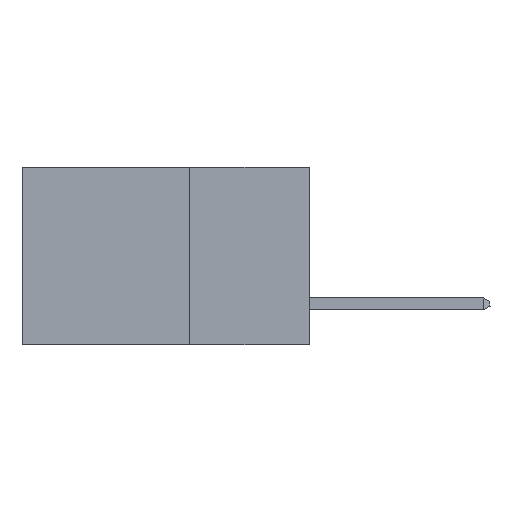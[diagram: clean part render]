
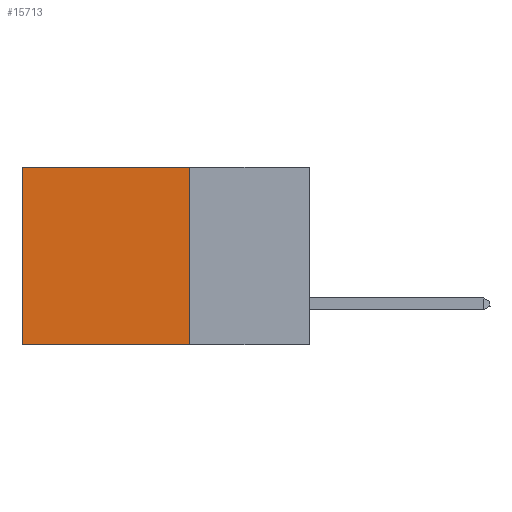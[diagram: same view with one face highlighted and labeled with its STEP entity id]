
A CAD part, left-side view. The second image highlights one B-rep face of the part: STEP entity #15713.
In plain terms, the highlighted planar face has unit normal (-1, 0, 0).
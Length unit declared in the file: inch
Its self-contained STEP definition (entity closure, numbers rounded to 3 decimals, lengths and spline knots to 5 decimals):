
#257 = VERTEX_POINT ( 'NONE', #1557 ) ;
#880 = LINE ( 'NONE', #9401, #15847 ) ;
#1231 = VERTEX_POINT ( 'NONE', #15142 ) ;
#1557 = CARTESIAN_POINT ( 'NONE',  ( 0.2875, 0.6, -0.37 ) ) ;
#1812 = CARTESIAN_POINT ( 'NONE',  ( 0.2875, 0.25, 0. ) ) ;
#1836 = CARTESIAN_POINT ( 'NONE',  ( 0.2875, 0.25, 0. ) ) ;
#1911 = VECTOR ( 'NONE', #5494, 39.37008 ) ;
#2403 = DIRECTION ( 'NONE',  ( 0., 1., 0. ) ) ;
#2406 = CARTESIAN_POINT ( 'NONE',  ( 0.2875, 0.6, 0. ) ) ;
#2424 = DIRECTION ( 'NONE',  ( 0., 0., -1. ) ) ;
#2433 = VECTOR ( 'NONE', #2403, 39.37008 ) ;
#3083 = EDGE_CURVE ( 'NONE', #3663, #257, #9772, .T. ) ;
#3663 = VERTEX_POINT ( 'NONE', #2406 ) ;
#4672 = CARTESIAN_POINT ( 'NONE',  ( 0.2875, 0.25, 0. ) ) ;
#5494 = DIRECTION ( 'NONE',  ( 0., 1., 0. ) ) ;
#5979 = DIRECTION ( 'NONE',  ( 1., 0., 0. ) ) ;
#6511 = FACE_OUTER_BOUND ( 'NONE', #6724, .T. ) ;
#6724 = EDGE_LOOP ( 'NONE', ( #13533, #13452, #14014, #13862 ) ) ;
#6954 = VECTOR ( 'NONE', #2424, 39.37008 ) ;
#7258 = DIRECTION ( 'NONE',  ( 0., 0., -1. ) ) ;
#8400 = AXIS2_PLACEMENT_3D ( 'NONE', #4672, #5979, #7258 ) ;
#9033 = EDGE_CURVE ( 'NONE', #11599, #1231, #880, .T. ) ;
#9194 = CARTESIAN_POINT ( 'NONE',  ( 0.2875, 0.25, -0.37 ) ) ;
#9261 = EDGE_CURVE ( 'NONE', #11599, #3663, #9694, .T. ) ;
#9401 = CARTESIAN_POINT ( 'NONE',  ( 0.2875, 0.25, 0. ) ) ;
#9694 = LINE ( 'NONE', #1836, #2433 ) ;
#9772 = LINE ( 'NONE', #10097, #6954 ) ;
#10097 = CARTESIAN_POINT ( 'NONE',  ( 0.2875, 0.6, 0. ) ) ;
#11599 = VERTEX_POINT ( 'NONE', #1812 ) ;
#12398 = PLANE ( 'NONE',  #8400 ) ;
#12483 = EDGE_CURVE ( 'NONE', #1231, #257, #15877, .T. ) ;
#13452 = ORIENTED_EDGE ( 'NONE', *, *, #12483, .F. ) ;
#13533 = ORIENTED_EDGE ( 'NONE', *, *, #3083, .T. ) ;
#13862 = ORIENTED_EDGE ( 'NONE', *, *, #9261, .T. ) ;
#14014 = ORIENTED_EDGE ( 'NONE', *, *, #9033, .F. ) ;
#15142 = CARTESIAN_POINT ( 'NONE',  ( 0.2875, 0.25, -0.37 ) ) ;
#15713 = ADVANCED_FACE ( 'NONE', ( #6511 ), #12398, .F. ) ;
#15771 = DIRECTION ( 'NONE',  ( 0., 0., -1. ) ) ;
#15847 = VECTOR ( 'NONE', #15771, 39.37008 ) ;
#15877 = LINE ( 'NONE', #9194, #1911 ) ;
